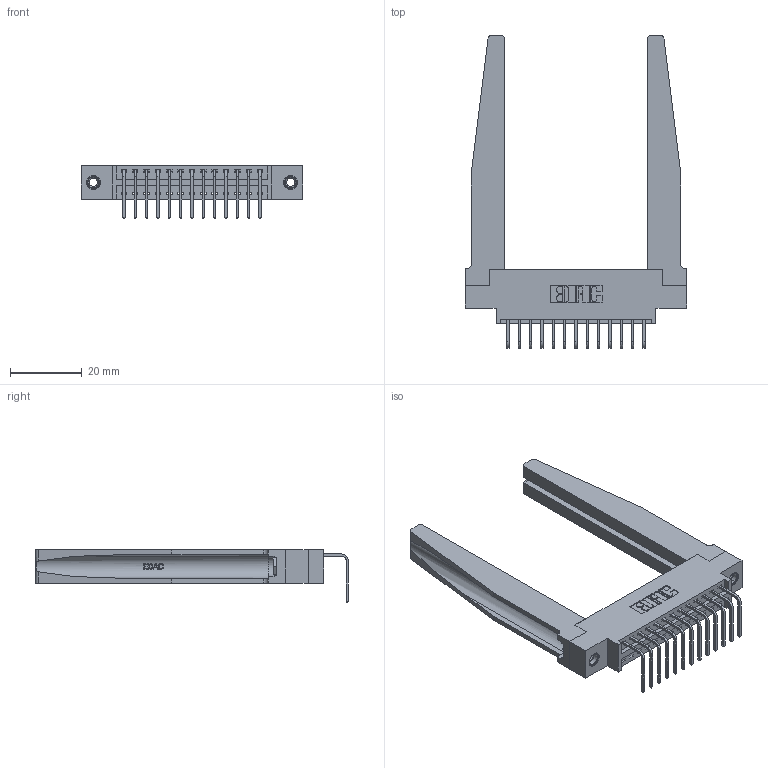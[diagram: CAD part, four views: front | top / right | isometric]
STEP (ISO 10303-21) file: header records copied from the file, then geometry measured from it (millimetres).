
FILE_DESCRIPTION (( 'STEP AP203' ), '1' );
FILE_NAME ('396-013-558-678.STEP', '2019-11-01T05:41:11', ( '' ), ( '' ), 'SwSTEP 2.0', 'SolidWorks 2016', '' );
FILE_SCHEMA (( 'CONFIG_CONTROL_DESIGN' ));
Length unit declared in the file: inch
Products named in the file (5): 346 Part_0.170 Offset - 0.156 Dia-TH; 345-292-001_558 Tail - 2; 346-220-078_345-220-078; 345-250-001_345-250-001-102; 396-013-558-678
Assembly tree (18 placements, depth 2):
  396-013-558-678
    346 Part_0.170 Offset - 0.156 Dia-TH
    345-292-001_558 Tail - 2  x13
    346-220-078_345-220-078  x2
    345-250-001_345-250-001-102  x2
Bounding box: 61.85 x 87.44 x 14.73 mm (x, y, z)
Volume: 12518.1 mm3; surface area: 13656.7 mm2
Topology: 18 solids, 18 shells, 1140 faces, 3315 edges, 2182 vertices
Faces by surface type: plane 768, cylinder 320, bspline 36, cone 12, torus 4
Entity records: 16936 total; most frequent: CARTESIAN_POINT 3826, ORIENTED_EDGE 2662, DIRECTION 2395, EDGE_CURVE 1331, VECTOR 1053, LINE 1053, VERTEX_POINT 880, AXIS2_PLACEMENT_3D 671
